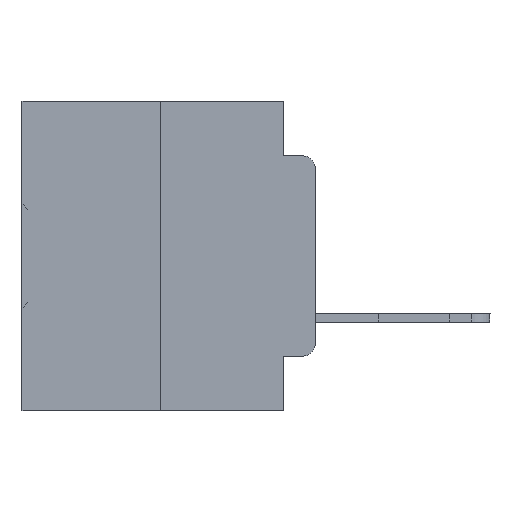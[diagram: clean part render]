
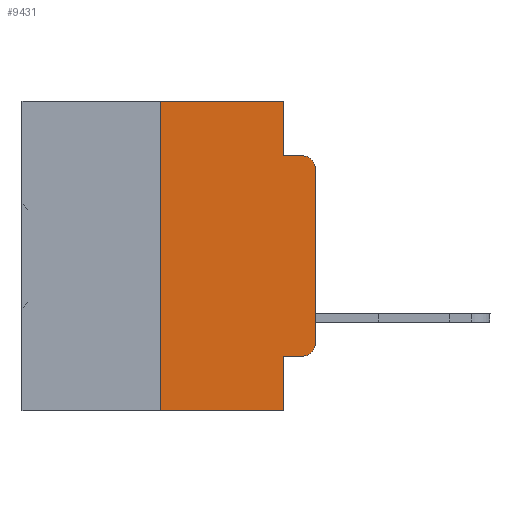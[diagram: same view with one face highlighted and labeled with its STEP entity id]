
A CAD part, left-side view. The second image highlights one B-rep face of the part: STEP entity #9431.
In plain terms, the highlighted planar face has unit normal (-1, 0, 0).
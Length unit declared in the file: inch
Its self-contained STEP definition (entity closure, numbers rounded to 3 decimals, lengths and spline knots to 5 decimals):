
#549 = CIRCLE ( 'NONE', #29342, 0.02 ) ;
#760 = CARTESIAN_POINT ( 'NONE',  ( 0., 0.25, 0. ) ) ;
#878 = DIRECTION ( 'NONE',  ( 0., 0., 1. ) ) ;
#1542 = ORIENTED_EDGE ( 'NONE', *, *, #2885, .T. ) ;
#2102 = CARTESIAN_POINT ( 'NONE',  ( 0., 0.473, 0. ) ) ;
#2817 = CARTESIAN_POINT ( 'NONE',  ( 0., 0.02, -0.4115 ) ) ;
#2870 = ORIENTED_EDGE ( 'NONE', *, *, #10743, .F. ) ;
#2885 = EDGE_CURVE ( 'NONE', #4862, #25919, #549, .T. ) ;
#2904 = LINE ( 'NONE', #760, #34821 ) ;
#3916 = VECTOR ( 'NONE', #26101, 39.37008 ) ;
#3964 = CARTESIAN_POINT ( 'NONE',  ( 0., 0.051, 0. ) ) ;
#4109 = EDGE_CURVE ( 'NONE', #7814, #4862, #29882, .T. ) ;
#4485 = CARTESIAN_POINT ( 'NONE',  ( 0., 0.02, -0.1085 ) ) ;
#4603 = DIRECTION ( 'NONE',  ( -1., 0., 0. ) ) ;
#4862 = VERTEX_POINT ( 'NONE', #20652 ) ;
#5700 = CARTESIAN_POINT ( 'NONE',  ( 0., 0.051, -0.4115 ) ) ;
#7185 = ORIENTED_EDGE ( 'NONE', *, *, #11534, .F. ) ;
#7378 = EDGE_CURVE ( 'NONE', #27493, #7814, #28829, .T. ) ;
#7496 = DIRECTION ( 'NONE',  ( 0., -1., 0. ) ) ;
#7579 = DIRECTION ( 'NONE',  ( 1., 0., 0. ) ) ;
#7814 = VERTEX_POINT ( 'NONE', #8493 ) ;
#8019 = CARTESIAN_POINT ( 'NONE',  ( 0., 0., 0. ) ) ;
#8218 = EDGE_CURVE ( 'NONE', #26413, #27606, #29639, .T. ) ;
#8493 = CARTESIAN_POINT ( 'NONE',  ( 0., 0., -0.3915 ) ) ;
#8904 = CARTESIAN_POINT ( 'NONE',  ( 0., 0.051, 0. ) ) ;
#9004 = LINE ( 'NONE', #20631, #3916 ) ;
#9308 = EDGE_LOOP ( 'NONE', ( #22656, #1542, #7185, #15570, #26869, #20459, #29416, #2870, #20681, #27088 ) ) ;
#9431 = ADVANCED_FACE ( 'NONE', ( #31682 ), #12786, .F. ) ;
#10082 = CARTESIAN_POINT ( 'NONE',  ( 0., 0.473, 0. ) ) ;
#10342 = CARTESIAN_POINT ( 'NONE',  ( 0., 0.051, -0.0885 ) ) ;
#10705 = DIRECTION ( 'NONE',  ( 0., -1., 0. ) ) ;
#10743 = EDGE_CURVE ( 'NONE', #25321, #31238, #9004, .T. ) ;
#11534 = EDGE_CURVE ( 'NONE', #18804, #25919, #29443, .T. ) ;
#11868 = AXIS2_PLACEMENT_3D ( 'NONE', #33655, #25480, #33426 ) ;
#12786 = PLANE ( 'NONE',  #18778 ) ;
#15160 = VECTOR ( 'NONE', #28947, 39.37008 ) ;
#15279 = DIRECTION ( 'NONE',  ( 0., -1., 0. ) ) ;
#15435 = CARTESIAN_POINT ( 'NONE',  ( 0., 0.051, -0.4115 ) ) ;
#15570 = ORIENTED_EDGE ( 'NONE', *, *, #15875, .F. ) ;
#15875 = EDGE_CURVE ( 'NONE', #27606, #18804, #30474, .T. ) ;
#17889 = CARTESIAN_POINT ( 'NONE',  ( 0., 0.473, -0.5 ) ) ;
#18288 = CARTESIAN_POINT ( 'NONE',  ( 0., 0.051, -0.0885 ) ) ;
#18291 = EDGE_CURVE ( 'NONE', #20648, #31238, #18396, .T. ) ;
#18396 = LINE ( 'NONE', #17889, #32013 ) ;
#18778 = AXIS2_PLACEMENT_3D ( 'NONE', #10082, #7579, #21378 ) ;
#18804 = VERTEX_POINT ( 'NONE', #18288 ) ;
#20456 = EDGE_CURVE ( 'NONE', #25321, #27493, #25077, .T. ) ;
#20459 = ORIENTED_EDGE ( 'NONE', *, *, #21492, .F. ) ;
#20631 = CARTESIAN_POINT ( 'NONE',  ( 0., 0.051, 0. ) ) ;
#20648 = VERTEX_POINT ( 'NONE', #25692 ) ;
#20652 = CARTESIAN_POINT ( 'NONE',  ( 0., 0., -0.1085 ) ) ;
#20681 = ORIENTED_EDGE ( 'NONE', *, *, #20456, .T. ) ;
#21378 = DIRECTION ( 'NONE',  ( 0., 0., -1. ) ) ;
#21492 = EDGE_CURVE ( 'NONE', #20648, #26413, #2904, .T. ) ;
#22656 = ORIENTED_EDGE ( 'NONE', *, *, #4109, .T. ) ;
#25077 = LINE ( 'NONE', #5700, #34009 ) ;
#25321 = VERTEX_POINT ( 'NONE', #15435 ) ;
#25480 = DIRECTION ( 'NONE',  ( -1., 0., 0. ) ) ;
#25692 = CARTESIAN_POINT ( 'NONE',  ( 0., 0.25, -0.5 ) ) ;
#25919 = VERTEX_POINT ( 'NONE', #30699 ) ;
#25972 = DIRECTION ( 'NONE',  ( 0., 0., -1. ) ) ;
#26101 = DIRECTION ( 'NONE',  ( 0., 0., -1. ) ) ;
#26413 = VERTEX_POINT ( 'NONE', #33793 ) ;
#26443 = CARTESIAN_POINT ( 'NONE',  ( 0., 0.051, -0.5 ) ) ;
#26869 = ORIENTED_EDGE ( 'NONE', *, *, #8218, .F. ) ;
#27088 = ORIENTED_EDGE ( 'NONE', *, *, #7378, .T. ) ;
#27493 = VERTEX_POINT ( 'NONE', #2817 ) ;
#27606 = VERTEX_POINT ( 'NONE', #3964 ) ;
#27695 = DIRECTION ( 'NONE',  ( 0., 0., -1. ) ) ;
#28829 = CIRCLE ( 'NONE', #11868, 0.02 ) ;
#28947 = DIRECTION ( 'NONE',  ( 0., -1., 0. ) ) ;
#29342 = AXIS2_PLACEMENT_3D ( 'NONE', #4485, #4603, #25972 ) ;
#29416 = ORIENTED_EDGE ( 'NONE', *, *, #18291, .T. ) ;
#29443 = LINE ( 'NONE', #10342, #30675 ) ;
#29639 = LINE ( 'NONE', #2102, #15160 ) ;
#29882 = LINE ( 'NONE', #8019, #30698 ) ;
#30474 = LINE ( 'NONE', #8904, #32213 ) ;
#30675 = VECTOR ( 'NONE', #7496, 39.37008 ) ;
#30698 = VECTOR ( 'NONE', #32514, 39.37008 ) ;
#30699 = CARTESIAN_POINT ( 'NONE',  ( 0., 0.02, -0.0885 ) ) ;
#31238 = VERTEX_POINT ( 'NONE', #26443 ) ;
#31682 = FACE_OUTER_BOUND ( 'NONE', #9308, .T. ) ;
#32013 = VECTOR ( 'NONE', #15279, 39.37008 ) ;
#32213 = VECTOR ( 'NONE', #27695, 39.37008 ) ;
#32514 = DIRECTION ( 'NONE',  ( 0., 0., 1. ) ) ;
#33426 = DIRECTION ( 'NONE',  ( 0., 0., -1. ) ) ;
#33655 = CARTESIAN_POINT ( 'NONE',  ( 0., 0.02, -0.3915 ) ) ;
#33793 = CARTESIAN_POINT ( 'NONE',  ( 0., 0.25, 0. ) ) ;
#34009 = VECTOR ( 'NONE', #10705, 39.37008 ) ;
#34821 = VECTOR ( 'NONE', #878, 39.37008 ) ;
